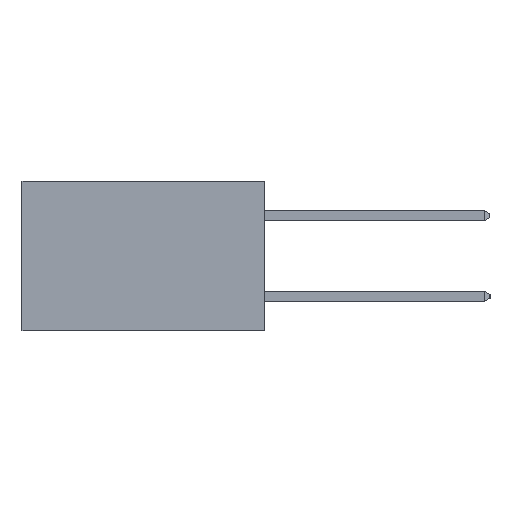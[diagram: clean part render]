
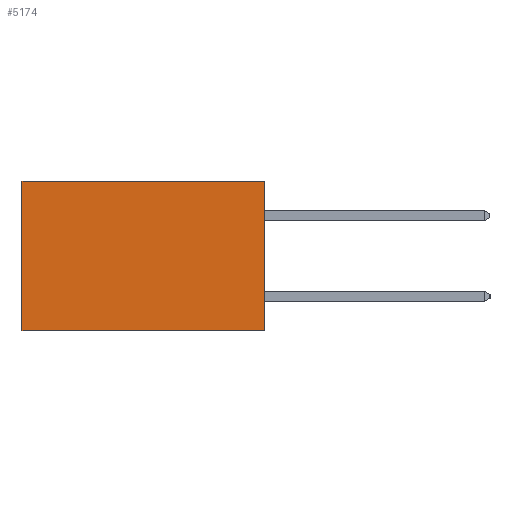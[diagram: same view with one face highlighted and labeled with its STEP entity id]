
A CAD part, left-side view. The second image highlights one B-rep face of the part: STEP entity #5174.
In plain terms, the highlighted planar face has unit normal (-1, 0, 0).
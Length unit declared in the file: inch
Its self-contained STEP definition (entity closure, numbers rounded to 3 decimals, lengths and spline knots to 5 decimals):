
#46 = ORIENTED_EDGE ( 'NONE', *, *, #10616, .F. ) ;
#378 = EDGE_LOOP ( 'NONE', ( #13184, #5254, #46, #3073 ) ) ;
#1789 = EDGE_CURVE ( 'NONE', #5953, #11198, #5683, .T. ) ;
#2004 = DIRECTION ( 'NONE',  ( 0., 0., -1. ) ) ;
#2110 = CARTESIAN_POINT ( 'NONE',  ( 0.2615, 0., -0.37 ) ) ;
#2125 = VECTOR ( 'NONE', #3413, 39.37008 ) ;
#2832 = VECTOR ( 'NONE', #4356, 39.37008 ) ;
#3073 = ORIENTED_EDGE ( 'NONE', *, *, #6709, .T. ) ;
#3303 = LINE ( 'NONE', #4252, #10733 ) ;
#3364 = CARTESIAN_POINT ( 'NONE',  ( 0.2615, 0., 0. ) ) ;
#3413 = DIRECTION ( 'NONE',  ( 0., 1., 0. ) ) ;
#4252 = CARTESIAN_POINT ( 'NONE',  ( 0.2615, 0., -0.37 ) ) ;
#4356 = DIRECTION ( 'NONE',  ( 0., 0., -1. ) ) ;
#4368 = DIRECTION ( 'NONE',  ( 0., 1., 0. ) ) ;
#4742 = CARTESIAN_POINT ( 'NONE',  ( 0.2615, 0., -0.37 ) ) ;
#5174 = ADVANCED_FACE ( 'NONE', ( #12241 ), #7732, .F. ) ;
#5254 = ORIENTED_EDGE ( 'NONE', *, *, #5463, .F. ) ;
#5397 = VERTEX_POINT ( 'NONE', #4742 ) ;
#5463 = EDGE_CURVE ( 'NONE', #5397, #11198, #3303, .T. ) ;
#5683 = LINE ( 'NONE', #8833, #2832 ) ;
#5847 = VECTOR ( 'NONE', #2004, 39.37008 ) ;
#5953 = VERTEX_POINT ( 'NONE', #11332 ) ;
#6189 = LINE ( 'NONE', #2110, #5847 ) ;
#6709 = EDGE_CURVE ( 'NONE', #9456, #5953, #10529, .T. ) ;
#7528 = DIRECTION ( 'NONE',  ( 0., 0., -1. ) ) ;
#7606 = DIRECTION ( 'NONE',  ( 1., 0., 0. ) ) ;
#7732 = PLANE ( 'NONE',  #9843 ) ;
#7747 = CARTESIAN_POINT ( 'NONE',  ( 0.2615, 0., -0.37 ) ) ;
#8833 = CARTESIAN_POINT ( 'NONE',  ( 0.2615, 0.6, -0.37 ) ) ;
#9456 = VERTEX_POINT ( 'NONE', #10838 ) ;
#9843 = AXIS2_PLACEMENT_3D ( 'NONE', #7747, #7606, #7528 ) ;
#10529 = LINE ( 'NONE', #3364, #2125 ) ;
#10616 = EDGE_CURVE ( 'NONE', #9456, #5397, #6189, .T. ) ;
#10733 = VECTOR ( 'NONE', #4368, 39.37008 ) ;
#10838 = CARTESIAN_POINT ( 'NONE',  ( 0.2615, 0., 0. ) ) ;
#11198 = VERTEX_POINT ( 'NONE', #11833 ) ;
#11332 = CARTESIAN_POINT ( 'NONE',  ( 0.2615, 0.6, 0. ) ) ;
#11833 = CARTESIAN_POINT ( 'NONE',  ( 0.2615, 0.6, -0.37 ) ) ;
#12241 = FACE_OUTER_BOUND ( 'NONE', #378, .T. ) ;
#13184 = ORIENTED_EDGE ( 'NONE', *, *, #1789, .T. ) ;
